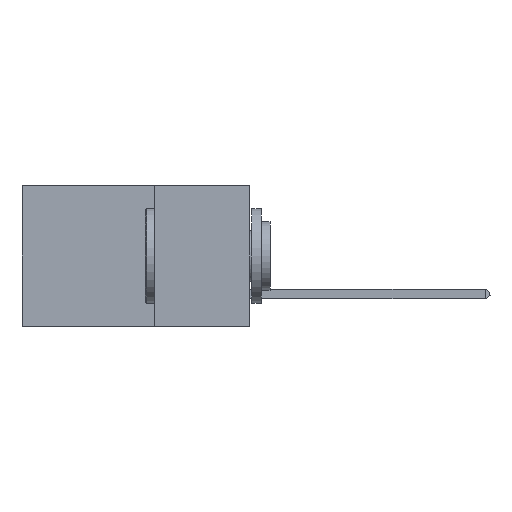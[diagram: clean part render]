
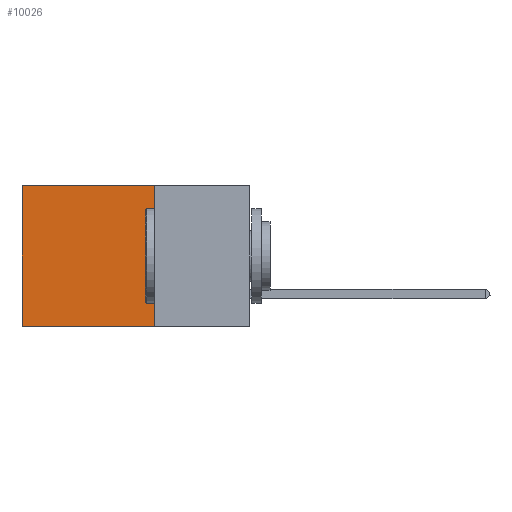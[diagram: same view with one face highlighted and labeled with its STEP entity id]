
A CAD part, left-side view. The second image highlights one B-rep face of the part: STEP entity #10026.
In plain terms, the highlighted planar face has unit normal (-1, 0, 0).
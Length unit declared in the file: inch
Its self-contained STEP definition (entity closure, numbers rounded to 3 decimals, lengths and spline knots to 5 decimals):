
#241 = CARTESIAN_POINT ( 'NONE',  ( 0.2875, 0.25, -0.37 ) ) ;
#983 = FACE_OUTER_BOUND ( 'NONE', #4616, .T. ) ;
#1270 = EDGE_CURVE ( 'NONE', #8573, #15847, #5849, .T. ) ;
#1357 = DIRECTION ( 'NONE',  ( 1., 0., 0. ) ) ;
#1380 = CARTESIAN_POINT ( 'NONE',  ( 0.2875, 0.25, 0. ) ) ;
#1480 = EDGE_CURVE ( 'NONE', #8573, #11972, #2490, .T. ) ;
#1584 = DIRECTION ( 'NONE',  ( 0., 1., 0. ) ) ;
#2490 = LINE ( 'NONE', #18088, #7397 ) ;
#3643 = LINE ( 'NONE', #6965, #8580 ) ;
#4247 = DIRECTION ( 'NONE',  ( 0., 0., -1. ) ) ;
#4616 = EDGE_LOOP ( 'NONE', ( #17907, #17734, #15326, #18401 ) ) ;
#5783 = VECTOR ( 'NONE', #10067, 39.37008 ) ;
#5849 = LINE ( 'NONE', #1380, #8769 ) ;
#5909 = CARTESIAN_POINT ( 'NONE',  ( 0.2875, 0.25, -0.37 ) ) ;
#6965 = CARTESIAN_POINT ( 'NONE',  ( 0.2875, 0.6, 0. ) ) ;
#7005 = VERTEX_POINT ( 'NONE', #16198 ) ;
#7397 = VECTOR ( 'NONE', #14984, 39.37008 ) ;
#7603 = DIRECTION ( 'NONE',  ( 0., 0., -1. ) ) ;
#8234 = CARTESIAN_POINT ( 'NONE',  ( 0.2875, 0.6, 0. ) ) ;
#8573 = VERTEX_POINT ( 'NONE', #10108 ) ;
#8580 = VECTOR ( 'NONE', #7603, 39.37008 ) ;
#8769 = VECTOR ( 'NONE', #1584, 39.37008 ) ;
#9040 = EDGE_CURVE ( 'NONE', #15847, #7005, #3643, .T. ) ;
#9476 = EDGE_CURVE ( 'NONE', #11972, #7005, #15505, .T. ) ;
#10026 = ADVANCED_FACE ( 'NONE', ( #983 ), #11312, .F. ) ;
#10067 = DIRECTION ( 'NONE',  ( 0., 1., 0. ) ) ;
#10108 = CARTESIAN_POINT ( 'NONE',  ( 0.2875, 0.25, 0. ) ) ;
#11312 = PLANE ( 'NONE',  #13406 ) ;
#11972 = VERTEX_POINT ( 'NONE', #5909 ) ;
#13406 = AXIS2_PLACEMENT_3D ( 'NONE', #15802, #1357, #4247 ) ;
#14984 = DIRECTION ( 'NONE',  ( 0., 0., -1. ) ) ;
#15326 = ORIENTED_EDGE ( 'NONE', *, *, #1480, .F. ) ;
#15505 = LINE ( 'NONE', #241, #5783 ) ;
#15802 = CARTESIAN_POINT ( 'NONE',  ( 0.2875, 0.25, 0. ) ) ;
#15847 = VERTEX_POINT ( 'NONE', #8234 ) ;
#16198 = CARTESIAN_POINT ( 'NONE',  ( 0.2875, 0.6, -0.37 ) ) ;
#17734 = ORIENTED_EDGE ( 'NONE', *, *, #9476, .F. ) ;
#17907 = ORIENTED_EDGE ( 'NONE', *, *, #9040, .T. ) ;
#18088 = CARTESIAN_POINT ( 'NONE',  ( 0.2875, 0.25, 0. ) ) ;
#18401 = ORIENTED_EDGE ( 'NONE', *, *, #1270, .T. ) ;
